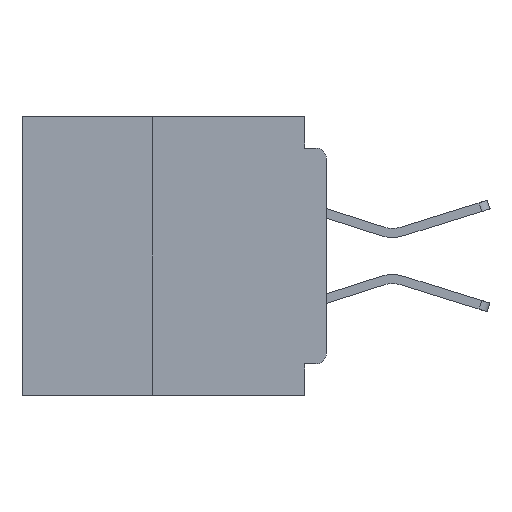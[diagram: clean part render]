
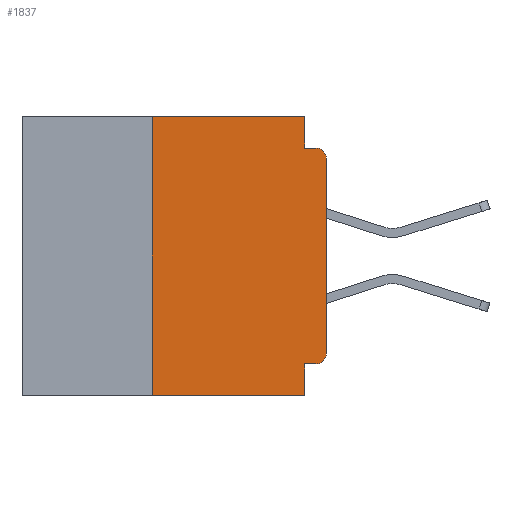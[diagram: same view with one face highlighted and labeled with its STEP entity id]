
A CAD part, left-side view. The second image highlights one B-rep face of the part: STEP entity #1837.
In plain terms, the highlighted planar face has unit normal (-1, 0, 0).
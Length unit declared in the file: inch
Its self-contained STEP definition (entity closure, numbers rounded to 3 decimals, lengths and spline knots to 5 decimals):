
#14 = CARTESIAN_POINT ( 'NONE',  ( 0., 0.25, 0. ) ) ;
#557 = CARTESIAN_POINT ( 'NONE',  ( 0., 0.015, -0.06 ) ) ;
#829 = VERTEX_POINT ( 'NONE', #34672 ) ;
#1532 = CARTESIAN_POINT ( 'NONE',  ( 0., 0.437, 0. ) ) ;
#1837 = ADVANCED_FACE ( 'NONE', ( #48683 ), #11823, .F. ) ;
#4835 = DIRECTION ( 'NONE',  ( 0., 0., -1. ) ) ;
#6765 = LINE ( 'NONE', #28968, #38445 ) ;
#7230 = CARTESIAN_POINT ( 'NONE',  ( 0., 0.031, 0. ) ) ;
#7995 = VERTEX_POINT ( 'NONE', #14 ) ;
#8280 = ORIENTED_EDGE ( 'NONE', *, *, #41556, .F. ) ;
#8314 = CARTESIAN_POINT ( 'NONE',  ( 0., 0.437, 0. ) ) ;
#9240 = VECTOR ( 'NONE', #52070, 39.37008 ) ;
#10739 = CARTESIAN_POINT ( 'NONE',  ( 0., 0.031, 0. ) ) ;
#11031 = CARTESIAN_POINT ( 'NONE',  ( 0., 0.25, -0.4 ) ) ;
#11033 = LINE ( 'NONE', #1532, #22022 ) ;
#11211 = CARTESIAN_POINT ( 'NONE',  ( 0., 0., -0.355 ) ) ;
#11412 = DIRECTION ( 'NONE',  ( 1., 0., 0. ) ) ;
#11685 = VECTOR ( 'NONE', #15353, 39.37008 ) ;
#11688 = VERTEX_POINT ( 'NONE', #10739 ) ;
#11823 = PLANE ( 'NONE',  #37235 ) ;
#12314 = DIRECTION ( 'NONE',  ( 0., 0., -1. ) ) ;
#12391 = EDGE_CURVE ( 'NONE', #22330, #13212, #44593, .T. ) ;
#12397 = EDGE_CURVE ( 'NONE', #11688, #829, #32388, .T. ) ;
#13212 = VERTEX_POINT ( 'NONE', #43654 ) ;
#15002 = ORIENTED_EDGE ( 'NONE', *, *, #46039, .F. ) ;
#15353 = DIRECTION ( 'NONE',  ( 0., 1., 0. ) ) ;
#16062 = CIRCLE ( 'NONE', #33807, 0.015 ) ;
#16909 = ORIENTED_EDGE ( 'NONE', *, *, #44533, .T. ) ;
#17736 = VERTEX_POINT ( 'NONE', #44197 ) ;
#17759 = EDGE_LOOP ( 'NONE', ( #53069, #26138, #8280, #46953, #24059, #44918, #28546, #15002, #29770, #16909 ) ) ;
#17829 = LINE ( 'NONE', #39467, #51920 ) ;
#18833 = EDGE_CURVE ( 'NONE', #35978, #17736, #36278, .T. ) ;
#19348 = DIRECTION ( 'NONE',  ( -1., 0., 0. ) ) ;
#22022 = VECTOR ( 'NONE', #34712, 39.37008 ) ;
#22330 = VERTEX_POINT ( 'NONE', #43903 ) ;
#22857 = EDGE_CURVE ( 'NONE', #7995, #11688, #11033, .T. ) ;
#22912 = DIRECTION ( 'NONE',  ( 0., -1., 0. ) ) ;
#24027 = VECTOR ( 'NONE', #32700, 39.37008 ) ;
#24059 = ORIENTED_EDGE ( 'NONE', *, *, #22857, .F. ) ;
#26138 = ORIENTED_EDGE ( 'NONE', *, *, #39042, .T. ) ;
#27003 = CIRCLE ( 'NONE', #28837, 0.015 ) ;
#28546 = ORIENTED_EDGE ( 'NONE', *, *, #42813, .T. ) ;
#28837 = AXIS2_PLACEMENT_3D ( 'NONE', #44023, #19348, #48128 ) ;
#28968 = CARTESIAN_POINT ( 'NONE',  ( 0., 0.031, -0.4 ) ) ;
#29624 = DIRECTION ( 'NONE',  ( -1., 0., 0. ) ) ;
#29770 = ORIENTED_EDGE ( 'NONE', *, *, #12391, .F. ) ;
#31257 = LINE ( 'NONE', #47960, #9240 ) ;
#32016 = DIRECTION ( 'NONE',  ( 0., 0., -1. ) ) ;
#32388 = LINE ( 'NONE', #7230, #42013 ) ;
#32700 = DIRECTION ( 'NONE',  ( 0., 0., 1. ) ) ;
#33807 = AXIS2_PLACEMENT_3D ( 'NONE', #557, #29624, #4835 ) ;
#34672 = CARTESIAN_POINT ( 'NONE',  ( 0., 0.031, -0.045 ) ) ;
#34712 = DIRECTION ( 'NONE',  ( 0., -1., 0. ) ) ;
#35019 = VERTEX_POINT ( 'NONE', #52311 ) ;
#35978 = VERTEX_POINT ( 'NONE', #53187 ) ;
#36278 = LINE ( 'NONE', #48996, #24027 ) ;
#37087 = CARTESIAN_POINT ( 'NONE',  ( 0., 0.015, -0.045 ) ) ;
#37235 = AXIS2_PLACEMENT_3D ( 'NONE', #8314, #11412, #38362 ) ;
#37582 = VECTOR ( 'NONE', #44047, 39.37008 ) ;
#38362 = DIRECTION ( 'NONE',  ( 0., 0., -1. ) ) ;
#38445 = VECTOR ( 'NONE', #12314, 39.37008 ) ;
#38845 = LINE ( 'NONE', #11031, #37582 ) ;
#39042 = EDGE_CURVE ( 'NONE', #17736, #44275, #16062, .T. ) ;
#39467 = CARTESIAN_POINT ( 'NONE',  ( 0., 0., -0.045 ) ) ;
#40774 = VERTEX_POINT ( 'NONE', #42020 ) ;
#41556 = EDGE_CURVE ( 'NONE', #829, #44275, #17829, .T. ) ;
#42013 = VECTOR ( 'NONE', #32016, 39.37008 ) ;
#42020 = CARTESIAN_POINT ( 'NONE',  ( 0., 0.25, -0.4 ) ) ;
#42813 = EDGE_CURVE ( 'NONE', #40774, #35019, #31257, .T. ) ;
#43654 = CARTESIAN_POINT ( 'NONE',  ( 0., 0.031, -0.355 ) ) ;
#43903 = CARTESIAN_POINT ( 'NONE',  ( 0., 0.015, -0.355 ) ) ;
#44023 = CARTESIAN_POINT ( 'NONE',  ( 0., 0.015, -0.34 ) ) ;
#44047 = DIRECTION ( 'NONE',  ( 0., 0., 1. ) ) ;
#44197 = CARTESIAN_POINT ( 'NONE',  ( 0., 0., -0.06 ) ) ;
#44275 = VERTEX_POINT ( 'NONE', #37087 ) ;
#44533 = EDGE_CURVE ( 'NONE', #22330, #35978, #27003, .T. ) ;
#44593 = LINE ( 'NONE', #11211, #11685 ) ;
#44918 = ORIENTED_EDGE ( 'NONE', *, *, #51332, .F. ) ;
#46039 = EDGE_CURVE ( 'NONE', #13212, #35019, #6765, .T. ) ;
#46953 = ORIENTED_EDGE ( 'NONE', *, *, #12397, .F. ) ;
#47960 = CARTESIAN_POINT ( 'NONE',  ( 0., 0.437, -0.4 ) ) ;
#48128 = DIRECTION ( 'NONE',  ( 0., 0., -1. ) ) ;
#48683 = FACE_OUTER_BOUND ( 'NONE', #17759, .T. ) ;
#48996 = CARTESIAN_POINT ( 'NONE',  ( 0., 0., 0. ) ) ;
#51332 = EDGE_CURVE ( 'NONE', #40774, #7995, #38845, .T. ) ;
#51920 = VECTOR ( 'NONE', #22912, 39.37008 ) ;
#52070 = DIRECTION ( 'NONE',  ( 0., -1., 0. ) ) ;
#52311 = CARTESIAN_POINT ( 'NONE',  ( 0., 0.031, -0.4 ) ) ;
#53069 = ORIENTED_EDGE ( 'NONE', *, *, #18833, .T. ) ;
#53187 = CARTESIAN_POINT ( 'NONE',  ( 0., 0., -0.34 ) ) ;
